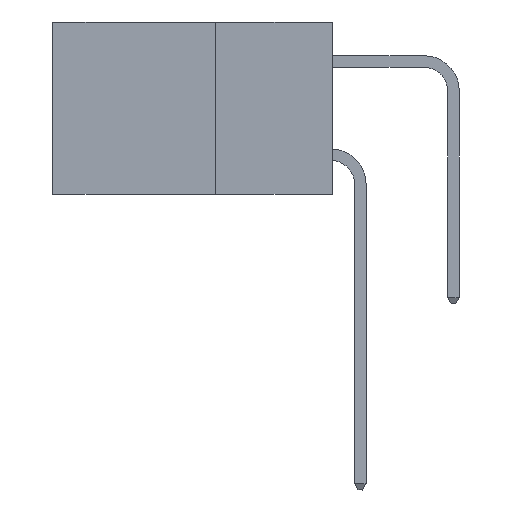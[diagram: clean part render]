
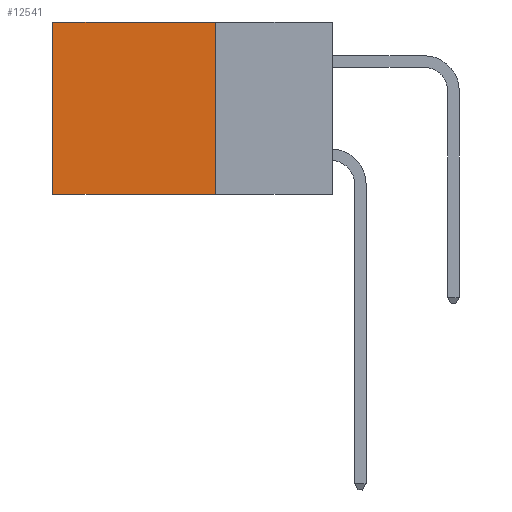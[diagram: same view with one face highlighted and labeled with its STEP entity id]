
A CAD part, left-side view. The second image highlights one B-rep face of the part: STEP entity #12541.
In plain terms, the highlighted planar face has unit normal (-1, 0, 0).
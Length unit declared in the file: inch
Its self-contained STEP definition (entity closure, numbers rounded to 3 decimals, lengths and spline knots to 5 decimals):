
#3131 = FACE_OUTER_BOUND ( 'NONE', #11352, .T. ) ;
#4310 = EDGE_CURVE ( 'NONE', #16036, #31694, #21951, .T. ) ;
#5733 = ORIENTED_EDGE ( 'NONE', *, *, #4310, .T. ) ;
#7664 = EDGE_CURVE ( 'NONE', #23970, #30574, #26182, .T. ) ;
#7959 = CARTESIAN_POINT ( 'NONE',  ( 0.298, 0.25, 0. ) ) ;
#8175 = CARTESIAN_POINT ( 'NONE',  ( 0.298, 0.25, 0. ) ) ;
#10643 = DIRECTION ( 'NONE',  ( 0., 0., -1. ) ) ;
#10858 = DIRECTION ( 'NONE',  ( 0., 1., 0. ) ) ;
#11352 = EDGE_LOOP ( 'NONE', ( #29798, #12902, #24772, #5733 ) ) ;
#11866 = CARTESIAN_POINT ( 'NONE',  ( 0.298, 0.6, -0.37 ) ) ;
#12114 = VECTOR ( 'NONE', #16928, 39.37008 ) ;
#12541 = ADVANCED_FACE ( 'NONE', ( #3131 ), #21097, .F. ) ;
#12902 = ORIENTED_EDGE ( 'NONE', *, *, #7664, .F. ) ;
#13916 = VECTOR ( 'NONE', #17107, 39.37008 ) ;
#14278 = CARTESIAN_POINT ( 'NONE',  ( 0.298, 0.6, 0. ) ) ;
#15435 = DIRECTION ( 'NONE',  ( 0., 0., -1. ) ) ;
#16036 = VERTEX_POINT ( 'NONE', #22511 ) ;
#16928 = DIRECTION ( 'NONE',  ( 0., 0., -1. ) ) ;
#17107 = DIRECTION ( 'NONE',  ( 0., 1., 0. ) ) ;
#18284 = EDGE_CURVE ( 'NONE', #31694, #30574, #33828, .T. ) ;
#21097 = PLANE ( 'NONE',  #31231 ) ;
#21129 = VECTOR ( 'NONE', #10858, 39.37008 ) ;
#21768 = VECTOR ( 'NONE', #15435, 39.37008 ) ;
#21951 = LINE ( 'NONE', #8175, #21129 ) ;
#21984 = EDGE_CURVE ( 'NONE', #16036, #23970, #28735, .T. ) ;
#22511 = CARTESIAN_POINT ( 'NONE',  ( 0.298, 0.25, 0. ) ) ;
#23646 = CARTESIAN_POINT ( 'NONE',  ( 0.298, 0.25, -0.37 ) ) ;
#23970 = VERTEX_POINT ( 'NONE', #23646 ) ;
#24772 = ORIENTED_EDGE ( 'NONE', *, *, #21984, .F. ) ;
#26182 = LINE ( 'NONE', #30157, #13916 ) ;
#26364 = DIRECTION ( 'NONE',  ( 1., 0., 0. ) ) ;
#26672 = CARTESIAN_POINT ( 'NONE',  ( 0.298, 0.6, 0. ) ) ;
#28735 = LINE ( 'NONE', #33724, #21768 ) ;
#29798 = ORIENTED_EDGE ( 'NONE', *, *, #18284, .T. ) ;
#30157 = CARTESIAN_POINT ( 'NONE',  ( 0.298, 0.25, -0.37 ) ) ;
#30574 = VERTEX_POINT ( 'NONE', #11866 ) ;
#31231 = AXIS2_PLACEMENT_3D ( 'NONE', #7959, #26364, #10643 ) ;
#31694 = VERTEX_POINT ( 'NONE', #26672 ) ;
#33724 = CARTESIAN_POINT ( 'NONE',  ( 0.298, 0.25, 0. ) ) ;
#33828 = LINE ( 'NONE', #14278, #12114 ) ;
